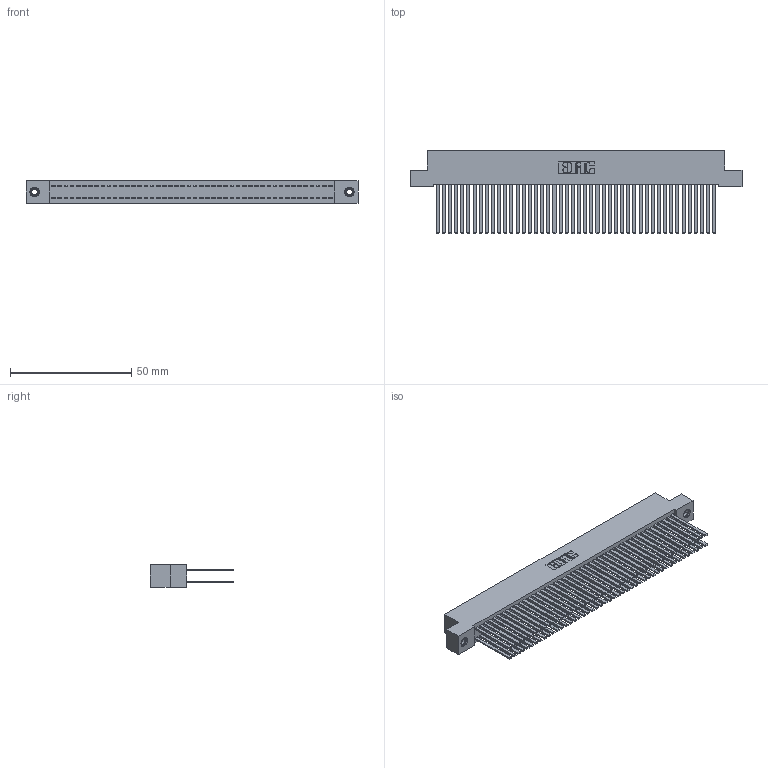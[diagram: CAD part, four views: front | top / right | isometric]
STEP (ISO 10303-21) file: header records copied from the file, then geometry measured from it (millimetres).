
FILE_DESCRIPTION (( 'STEP AP203' ), '1' );
FILE_NAME ('342-092-544-207.STEP', '2019-10-04T14:57:48', ( '' ), ( '' ), 'SwSTEP 2.0', 'SolidWorks 2016', '' );
FILE_SCHEMA (( 'CONFIG_CONTROL_DESIGN' ));
Length unit declared in the file: inch
Products named in the file (4): 342-092-544-207; 342 Part_TI; 345-292-001_345-293-144; 345-250-001_345-250-005-103
Assembly tree (95 placements, depth 2):
  342-092-544-207
    342 Part_TI
    345-292-001_345-293-144  x92
    345-250-001_345-250-005-103  x2
Bounding box: 137.16 x 34.3 x 9.4 mm (x, y, z)
Volume: 13619.7 mm3; surface area: 25865.4 mm2
Topology: 95 solids, 95 shells, 4402 faces, 13039 edges, 8562 vertices
Faces by surface type: plane 3042, cylinder 1344, cone 12, torus 4
Entity records: 29946 total; most frequent: CARTESIAN_POINT 4937, ORIENTED_EDGE 4866, DIRECTION 4239, EDGE_CURVE 2433, LINE 2289, VECTOR 2289, VERTEX_POINT 1616, AXIS2_PLACEMENT_3D 975
